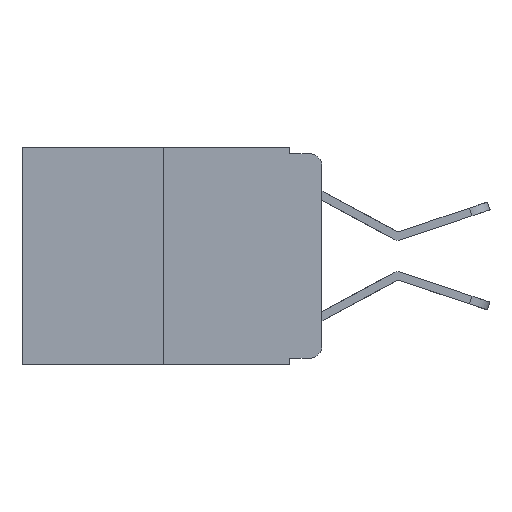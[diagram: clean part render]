
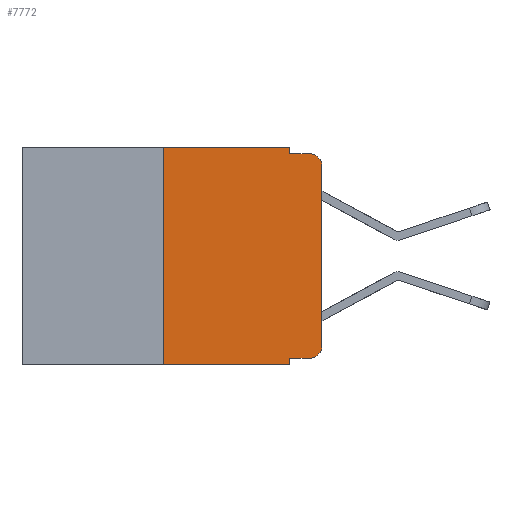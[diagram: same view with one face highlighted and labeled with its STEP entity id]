
A CAD part, left-side view. The second image highlights one B-rep face of the part: STEP entity #7772.
In plain terms, the highlighted planar face has unit normal (-1, 0, 0).
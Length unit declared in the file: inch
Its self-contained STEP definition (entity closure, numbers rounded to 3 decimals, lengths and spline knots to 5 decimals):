
#357 = ORIENTED_EDGE ( 'NONE', *, *, #436, .F. ) ;
#436 = EDGE_CURVE ( 'NONE', #9169, #19254, #23229, .T. ) ;
#438 = VECTOR ( 'NONE', #23941, 39.37008 ) ;
#716 = VERTEX_POINT ( 'NONE', #4178 ) ;
#856 = EDGE_CURVE ( 'NONE', #7140, #19434, #24387, .T. ) ;
#1117 = PLANE ( 'NONE',  #12884 ) ;
#1154 = CARTESIAN_POINT ( 'NONE',  ( 0., 0.25, 0. ) ) ;
#1545 = CARTESIAN_POINT ( 'NONE',  ( 0., 0.051, -0.333 ) ) ;
#2057 = AXIS2_PLACEMENT_3D ( 'NONE', #2232, #8821, #24785 ) ;
#2232 = CARTESIAN_POINT ( 'NONE',  ( 0., 0.02, -0.313 ) ) ;
#2372 = DIRECTION ( 'NONE',  ( 0., 0., 1. ) ) ;
#2553 = CARTESIAN_POINT ( 'NONE',  ( 0., 0.25, -0.343 ) ) ;
#2845 = CARTESIAN_POINT ( 'NONE',  ( 0., 0.473, -0.343 ) ) ;
#3143 = ORIENTED_EDGE ( 'NONE', *, *, #15920, .T. ) ;
#3249 = CARTESIAN_POINT ( 'NONE',  ( 0., 0.473, 0. ) ) ;
#3400 = VECTOR ( 'NONE', #21715, 39.37008 ) ;
#4178 = CARTESIAN_POINT ( 'NONE',  ( 0., 0., -0.03 ) ) ;
#5112 = FACE_OUTER_BOUND ( 'NONE', #21312, .T. ) ;
#5321 = DIRECTION ( 'NONE',  ( 1., 0., 0. ) ) ;
#5608 = ORIENTED_EDGE ( 'NONE', *, *, #24367, .F. ) ;
#5965 = LINE ( 'NONE', #20214, #16340 ) ;
#6366 = CARTESIAN_POINT ( 'NONE',  ( 0., 0.051, 0. ) ) ;
#6519 = VECTOR ( 'NONE', #20656, 39.37008 ) ;
#7140 = VERTEX_POINT ( 'NONE', #24803 ) ;
#7366 = ORIENTED_EDGE ( 'NONE', *, *, #23094, .F. ) ;
#7648 = VECTOR ( 'NONE', #23428, 39.37008 ) ;
#7772 = ADVANCED_FACE ( 'NONE', ( #5112 ), #1117, .F. ) ;
#7824 = CARTESIAN_POINT ( 'NONE',  ( 0., 0.051, -0.01 ) ) ;
#7902 = CARTESIAN_POINT ( 'NONE',  ( 0., 0.02, -0.03 ) ) ;
#8805 = VECTOR ( 'NONE', #11775, 39.37008 ) ;
#8821 = DIRECTION ( 'NONE',  ( -1., 0., 0. ) ) ;
#9169 = VERTEX_POINT ( 'NONE', #13952 ) ;
#9356 = VERTEX_POINT ( 'NONE', #2553 ) ;
#9544 = EDGE_CURVE ( 'NONE', #9356, #9169, #15420, .T. ) ;
#9894 = DIRECTION ( 'NONE',  ( 0., 0., -1. ) ) ;
#9968 = CIRCLE ( 'NONE', #14608, 0.02 ) ;
#11635 = ORIENTED_EDGE ( 'NONE', *, *, #14747, .F. ) ;
#11775 = DIRECTION ( 'NONE',  ( 0., -1., 0. ) ) ;
#11942 = LINE ( 'NONE', #1545, #21135 ) ;
#12017 = CARTESIAN_POINT ( 'NONE',  ( 0., 0.02, -0.01 ) ) ;
#12772 = ORIENTED_EDGE ( 'NONE', *, *, #15228, .T. ) ;
#12884 = AXIS2_PLACEMENT_3D ( 'NONE', #3249, #5321, #19055 ) ;
#12934 = CARTESIAN_POINT ( 'NONE',  ( 0., 0.051, 0. ) ) ;
#13162 = DIRECTION ( 'NONE',  ( 0., 0., 1. ) ) ;
#13677 = ORIENTED_EDGE ( 'NONE', *, *, #20034, .T. ) ;
#13683 = CARTESIAN_POINT ( 'NONE',  ( 0., 0.051, -0.333 ) ) ;
#13952 = CARTESIAN_POINT ( 'NONE',  ( 0., 0.25, 0. ) ) ;
#14218 = ORIENTED_EDGE ( 'NONE', *, *, #9544, .F. ) ;
#14391 = ORIENTED_EDGE ( 'NONE', *, *, #856, .T. ) ;
#14608 = AXIS2_PLACEMENT_3D ( 'NONE', #7902, #21582, #9894 ) ;
#14627 = CARTESIAN_POINT ( 'NONE',  ( 0., 0.051, -0.01 ) ) ;
#14747 = EDGE_CURVE ( 'NONE', #24265, #20724, #16354, .T. ) ;
#15228 = EDGE_CURVE ( 'NONE', #716, #23168, #9968, .T. ) ;
#15420 = LINE ( 'NONE', #1154, #25175 ) ;
#15446 = DIRECTION ( 'NONE',  ( 0., -1., 0. ) ) ;
#15530 = EDGE_CURVE ( 'NONE', #9356, #20724, #22143, .T. ) ;
#15869 = CARTESIAN_POINT ( 'NONE',  ( 0., 0.051, 0. ) ) ;
#15920 = EDGE_CURVE ( 'NONE', #19434, #716, #5965, .T. ) ;
#16340 = VECTOR ( 'NONE', #2372, 39.37008 ) ;
#16354 = LINE ( 'NONE', #6366, #438 ) ;
#17457 = CARTESIAN_POINT ( 'NONE',  ( 0., 0., -0.313 ) ) ;
#18587 = ORIENTED_EDGE ( 'NONE', *, *, #15530, .T. ) ;
#19055 = DIRECTION ( 'NONE',  ( 0., 0., -1. ) ) ;
#19162 = LINE ( 'NONE', #15869, #3400 ) ;
#19254 = VERTEX_POINT ( 'NONE', #12934 ) ;
#19434 = VERTEX_POINT ( 'NONE', #17457 ) ;
#19511 = CARTESIAN_POINT ( 'NONE',  ( 0., 0.051, -0.343 ) ) ;
#20034 = EDGE_CURVE ( 'NONE', #24265, #7140, #11942, .T. ) ;
#20214 = CARTESIAN_POINT ( 'NONE',  ( 0., 0., 0. ) ) ;
#20656 = DIRECTION ( 'NONE',  ( 0., -1., 0. ) ) ;
#20724 = VERTEX_POINT ( 'NONE', #19511 ) ;
#21135 = VECTOR ( 'NONE', #15446, 39.37008 ) ;
#21312 = EDGE_LOOP ( 'NONE', ( #3143, #12772, #7366, #5608, #357, #14218, #18587, #11635, #13677, #14391 ) ) ;
#21543 = VERTEX_POINT ( 'NONE', #14627 ) ;
#21582 = DIRECTION ( 'NONE',  ( -1., 0., 0. ) ) ;
#21715 = DIRECTION ( 'NONE',  ( 0., 0., -1. ) ) ;
#22143 = LINE ( 'NONE', #2845, #6519 ) ;
#23094 = EDGE_CURVE ( 'NONE', #21543, #23168, #24343, .T. ) ;
#23168 = VERTEX_POINT ( 'NONE', #12017 ) ;
#23229 = LINE ( 'NONE', #23289, #7648 ) ;
#23289 = CARTESIAN_POINT ( 'NONE',  ( 0., 0.473, 0. ) ) ;
#23428 = DIRECTION ( 'NONE',  ( 0., -1., 0. ) ) ;
#23941 = DIRECTION ( 'NONE',  ( 0., 0., -1. ) ) ;
#24265 = VERTEX_POINT ( 'NONE', #13683 ) ;
#24343 = LINE ( 'NONE', #7824, #8805 ) ;
#24367 = EDGE_CURVE ( 'NONE', #19254, #21543, #19162, .T. ) ;
#24387 = CIRCLE ( 'NONE', #2057, 0.02 ) ;
#24785 = DIRECTION ( 'NONE',  ( 0., 0., -1. ) ) ;
#24803 = CARTESIAN_POINT ( 'NONE',  ( 0., 0.02, -0.333 ) ) ;
#25175 = VECTOR ( 'NONE', #13162, 39.37008 ) ;
